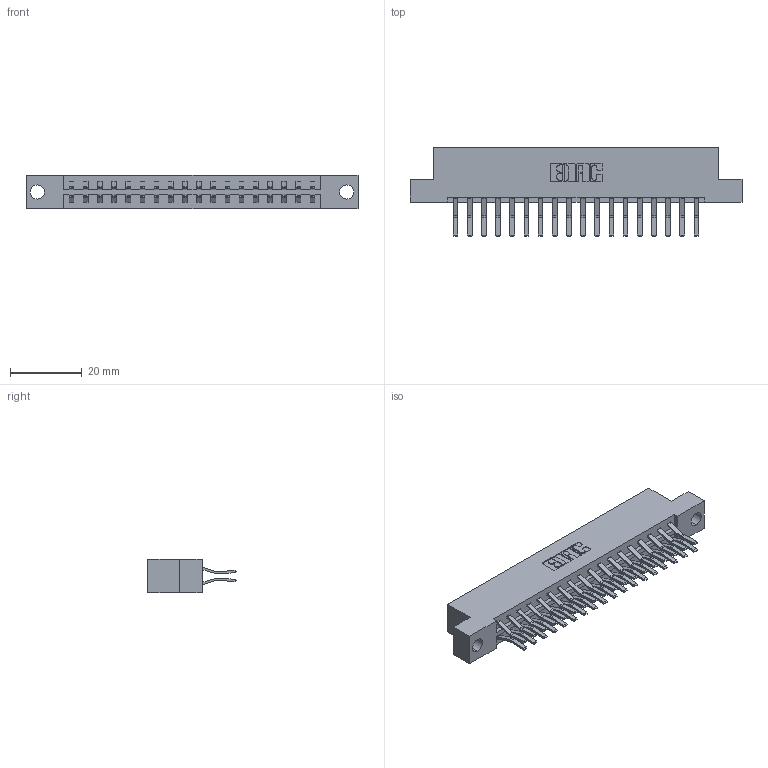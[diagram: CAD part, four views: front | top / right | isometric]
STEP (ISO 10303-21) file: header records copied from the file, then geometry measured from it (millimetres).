
FILE_DESCRIPTION (( 'STEP AP203' ), '1' );
FILE_NAME ('833-036-560-204.STEP', '2020-06-03T04:24:39', ( '' ), ( '' ), 'SwSTEP 2.0', 'SolidWorks 2020', '' );
FILE_SCHEMA (( 'CONFIG_CONTROL_DESIGN' ));
Length unit declared in the file: inch
Products named in the file (3): 833-036-560-204; 345-292-001_560 Tail; 833 Part_Flush - .156 Dia - TH
Assembly tree (37 placements, depth 2):
  833-036-560-204
    833 Part_Flush - .156 Dia - TH
    345-292-001_560 Tail  x36
Bounding box: 92.86 x 24.78 x 9.4 mm (x, y, z)
Volume: 9404.4 mm3; surface area: 11333 mm2
Topology: 37 solids, 37 shells, 2058 faces, 6107 edges, 4022 vertices
Faces by surface type: plane 1366, cylinder 692
Entity records: 14775 total; most frequent: CARTESIAN_POINT 2478, ORIENTED_EDGE 2414, DIRECTION 2163, EDGE_CURVE 1207, VECTOR 1075, LINE 1075, VERTEX_POINT 802, AXIS2_PLACEMENT_3D 544
